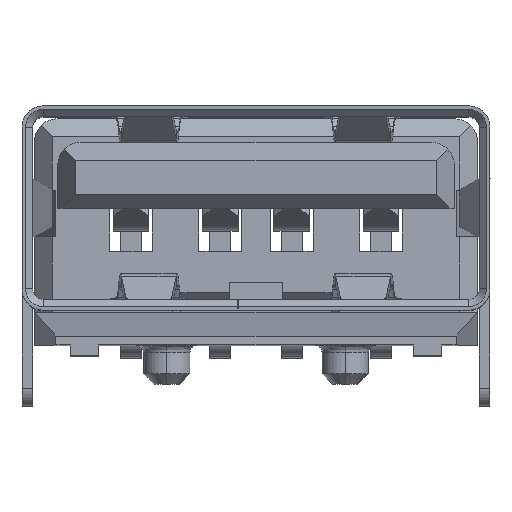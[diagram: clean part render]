
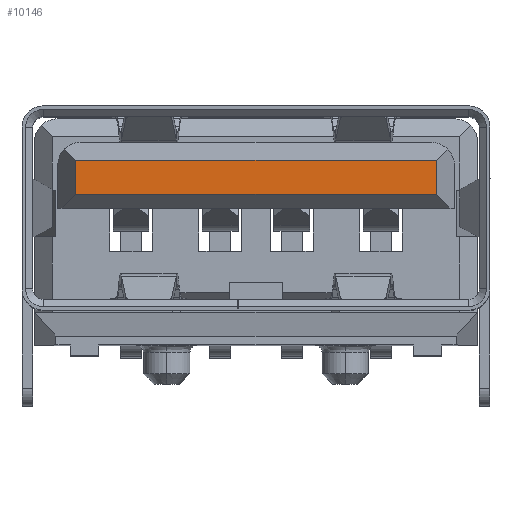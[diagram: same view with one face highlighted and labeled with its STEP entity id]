
A CAD part, top view. The second image highlights one B-rep face of the part: STEP entity #10146.
In plain terms, the highlighted planar face has unit normal (0, 0, 1).
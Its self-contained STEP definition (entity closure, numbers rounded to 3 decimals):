
#138 = LINE ( 'NONE', #15423, #17291 ) ;
#184 = DIRECTION ( 'NONE',  ( -1., 0., 0. ) ) ;
#1913 = AXIS2_PLACEMENT_3D ( 'NONE', #14825, #13285, #184 ) ;
#1928 = PLANE ( 'NONE',  #1913 ) ;
#2229 = VERTEX_POINT ( 'NONE', #20444 ) ;
#3796 = VECTOR ( 'NONE', #14686, 1000. ) ;
#4716 = LINE ( 'NONE', #13006, #14255 ) ;
#5504 = ORIENTED_EDGE ( 'NONE', *, *, #15956, .T. ) ;
#6040 = CARTESIAN_POINT ( 'NONE',  ( -5.05, 0.38, 8.38 ) ) ;
#8155 = FACE_OUTER_BOUND ( 'NONE', #17972, .T. ) ;
#8375 = VERTEX_POINT ( 'NONE', #20663 ) ;
#8612 = LINE ( 'NONE', #16909, #14101 ) ;
#9780 = EDGE_CURVE ( 'NONE', #11770, #8375, #8612, .T. ) ;
#10146 = ADVANCED_FACE ( 'NONE', ( #8155 ), #1928, .F. ) ;
#11453 = EDGE_CURVE ( 'NONE', #8375, #2229, #138, .T. ) ;
#11770 = VERTEX_POINT ( 'NONE', #16283 ) ;
#13006 = CARTESIAN_POINT ( 'NONE',  ( 4.91, 0.38, 8.38 ) ) ;
#13285 = DIRECTION ( 'NONE',  ( 0., 0., -1. ) ) ;
#14023 = EDGE_CURVE ( 'NONE', #11770, #17586, #4716, .T. ) ;
#14101 = VECTOR ( 'NONE', #15175, 1000. ) ;
#14255 = VECTOR ( 'NONE', #17943, 1000. ) ;
#14432 = ORIENTED_EDGE ( 'NONE', *, *, #14023, .F. ) ;
#14686 = DIRECTION ( 'NONE',  ( 0., -1., 0. ) ) ;
#14825 = CARTESIAN_POINT ( 'NONE',  ( 4.91, 1.2, 8.38 ) ) ;
#15175 = DIRECTION ( 'NONE',  ( 0., 1., 0. ) ) ;
#15423 = CARTESIAN_POINT ( 'NONE',  ( -5.55, 1.34, 8.38 ) ) ;
#15956 = EDGE_CURVE ( 'NONE', #2229, #17586, #17861, .T. ) ;
#16283 = CARTESIAN_POINT ( 'NONE',  ( 5.05, 0.38, 8.38 ) ) ;
#16909 = CARTESIAN_POINT ( 'NONE',  ( 5.05, -6.54, 8.38 ) ) ;
#17048 = DIRECTION ( 'NONE',  ( -1., 0., 0. ) ) ;
#17291 = VECTOR ( 'NONE', #17048, 1000. ) ;
#17586 = VERTEX_POINT ( 'NONE', #6040 ) ;
#17861 = LINE ( 'NONE', #18081, #3796 ) ;
#17943 = DIRECTION ( 'NONE',  ( -1., 0., 0. ) ) ;
#17972 = EDGE_LOOP ( 'NONE', ( #19407, #5504, #14432, #18749 ) ) ;
#18081 = CARTESIAN_POINT ( 'NONE',  ( -5.05, -6.54, 8.38 ) ) ;
#18749 = ORIENTED_EDGE ( 'NONE', *, *, #9780, .T. ) ;
#19407 = ORIENTED_EDGE ( 'NONE', *, *, #11453, .T. ) ;
#20444 = CARTESIAN_POINT ( 'NONE',  ( -5.05, 1.34, 8.38 ) ) ;
#20663 = CARTESIAN_POINT ( 'NONE',  ( 5.05, 1.34, 8.38 ) ) ;
